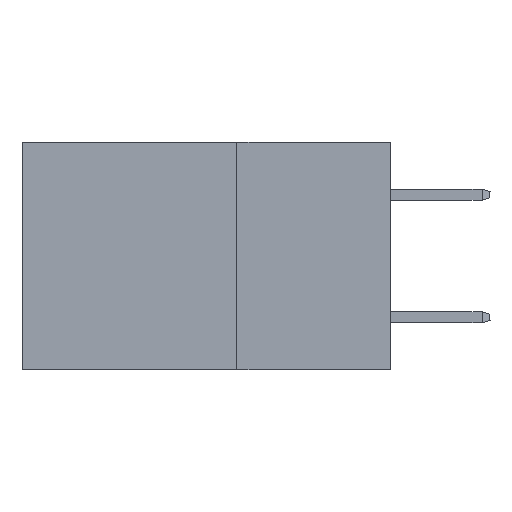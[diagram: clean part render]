
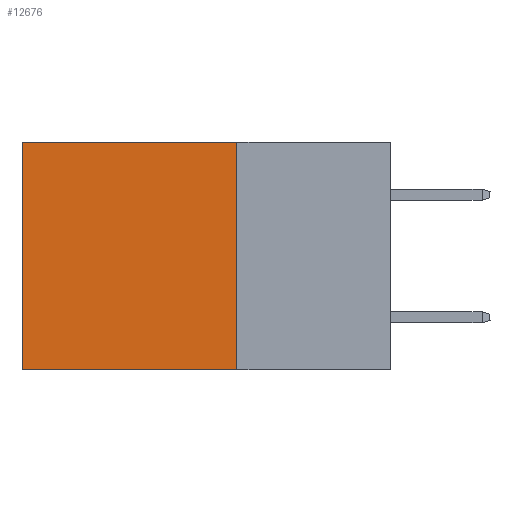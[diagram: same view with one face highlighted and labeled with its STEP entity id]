
A CAD part, left-side view. The second image highlights one B-rep face of the part: STEP entity #12676.
In plain terms, the highlighted planar face has unit normal (-1, 0, 0).
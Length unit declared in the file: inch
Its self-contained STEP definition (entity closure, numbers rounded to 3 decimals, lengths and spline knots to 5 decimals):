
#150 = CARTESIAN_POINT ( 'NONE',  ( 0.2875, 0.25, 0. ) ) ;
#2733 = DIRECTION ( 'NONE',  ( 0., 1., 0. ) ) ;
#3959 = VERTEX_POINT ( 'NONE', #20933 ) ;
#4258 = LINE ( 'NONE', #13848, #12614 ) ;
#7013 = ORIENTED_EDGE ( 'NONE', *, *, #23928, .T. ) ;
#7849 = VERTEX_POINT ( 'NONE', #8327 ) ;
#8327 = CARTESIAN_POINT ( 'NONE',  ( 0.2875, 0.6, -0.37 ) ) ;
#10137 = CARTESIAN_POINT ( 'NONE',  ( 0.2875, 0.6, 0. ) ) ;
#11485 = DIRECTION ( 'NONE',  ( 0., 1., 0. ) ) ;
#11493 = VECTOR ( 'NONE', #17790, 39.37008 ) ;
#12061 = EDGE_CURVE ( 'NONE', #24511, #3959, #25453, .T. ) ;
#12337 = LINE ( 'NONE', #10137, #15128 ) ;
#12614 = VECTOR ( 'NONE', #11485, 39.37008 ) ;
#12676 = ADVANCED_FACE ( 'NONE', ( #29830 ), #17965, .F. ) ;
#13581 = AXIS2_PLACEMENT_3D ( 'NONE', #30813, #25789, #25892 ) ;
#13610 = CARTESIAN_POINT ( 'NONE',  ( 0.2875, 0.6, 0. ) ) ;
#13848 = CARTESIAN_POINT ( 'NONE',  ( 0.2875, 0.25, 0. ) ) ;
#15108 = EDGE_LOOP ( 'NONE', ( #20879, #16225, #26489, #7013 ) ) ;
#15128 = VECTOR ( 'NONE', #25280, 39.37008 ) ;
#16225 = ORIENTED_EDGE ( 'NONE', *, *, #29184, .F. ) ;
#17790 = DIRECTION ( 'NONE',  ( 0., 0., -1. ) ) ;
#17965 = PLANE ( 'NONE',  #13581 ) ;
#18089 = VECTOR ( 'NONE', #2733, 39.37008 ) ;
#18207 = CARTESIAN_POINT ( 'NONE',  ( 0.2875, 0.25, -0.37 ) ) ;
#20879 = ORIENTED_EDGE ( 'NONE', *, *, #32201, .T. ) ;
#20933 = CARTESIAN_POINT ( 'NONE',  ( 0.2875, 0.25, -0.37 ) ) ;
#23822 = CARTESIAN_POINT ( 'NONE',  ( 0.2875, 0.25, 0. ) ) ;
#23928 = EDGE_CURVE ( 'NONE', #24511, #24557, #4258, .T. ) ;
#24511 = VERTEX_POINT ( 'NONE', #23822 ) ;
#24557 = VERTEX_POINT ( 'NONE', #13610 ) ;
#25280 = DIRECTION ( 'NONE',  ( 0., 0., -1. ) ) ;
#25453 = LINE ( 'NONE', #150, #11493 ) ;
#25789 = DIRECTION ( 'NONE',  ( 1., 0., 0. ) ) ;
#25892 = DIRECTION ( 'NONE',  ( 0., 0., -1. ) ) ;
#26489 = ORIENTED_EDGE ( 'NONE', *, *, #12061, .F. ) ;
#27675 = LINE ( 'NONE', #18207, #18089 ) ;
#29184 = EDGE_CURVE ( 'NONE', #3959, #7849, #27675, .T. ) ;
#29830 = FACE_OUTER_BOUND ( 'NONE', #15108, .T. ) ;
#30813 = CARTESIAN_POINT ( 'NONE',  ( 0.2875, 0.25, 0. ) ) ;
#32201 = EDGE_CURVE ( 'NONE', #24557, #7849, #12337, .T. ) ;
